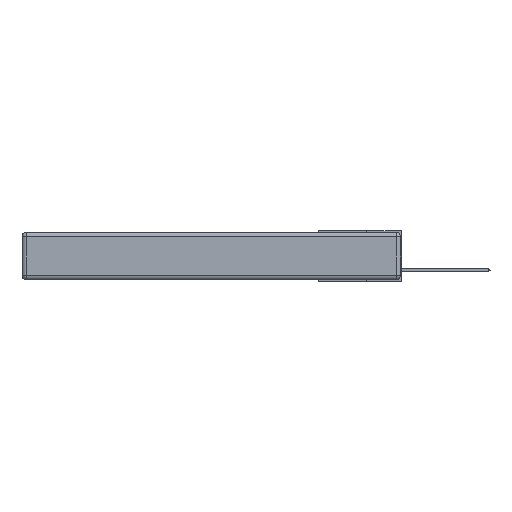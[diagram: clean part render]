
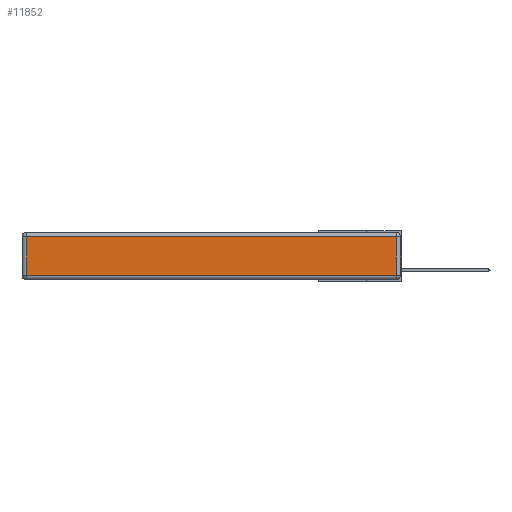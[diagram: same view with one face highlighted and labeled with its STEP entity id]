
A CAD part, left-side view. The second image highlights one B-rep face of the part: STEP entity #11852.
In plain terms, the highlighted planar face has unit normal (-1, 0, 0).
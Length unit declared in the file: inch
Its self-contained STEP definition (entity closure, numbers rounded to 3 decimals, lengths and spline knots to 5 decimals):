
#1438 = DIRECTION ( 'NONE',  ( -1., 0., 0. ) ) ;
#1815 = CARTESIAN_POINT ( 'NONE',  ( 0., 0.03, -0.03 ) ) ;
#3836 = CARTESIAN_POINT ( 'NONE',  ( 0., 2.72, -0.03 ) ) ;
#4516 = AXIS2_PLACEMENT_3D ( 'NONE', #21869, #1438, #6058 ) ;
#5223 = VECTOR ( 'NONE', #24640, 39.37008 ) ;
#5563 = VECTOR ( 'NONE', #8861, 39.37008 ) ;
#6058 = DIRECTION ( 'NONE',  ( 0., 0., 1. ) ) ;
#6269 = EDGE_CURVE ( 'NONE', #11951, #9548, #9448, .T. ) ;
#7486 = EDGE_CURVE ( 'NONE', #9548, #22008, #10480, .T. ) ;
#8087 = VERTEX_POINT ( 'NONE', #26164 ) ;
#8861 = DIRECTION ( 'NONE',  ( 0., -1., 0. ) ) ;
#9054 = CARTESIAN_POINT ( 'NONE',  ( 0., 2.75, -0.03 ) ) ;
#9448 = LINE ( 'NONE', #9054, #5223 ) ;
#9548 = VERTEX_POINT ( 'NONE', #3836 ) ;
#9661 = DIRECTION ( 'NONE',  ( 0., 0., 1. ) ) ;
#10480 = LINE ( 'NONE', #14195, #13611 ) ;
#11553 = LINE ( 'NONE', #27407, #26980 ) ;
#11852 = ADVANCED_FACE ( 'NONE', ( #28037 ), #19731, .T. ) ;
#11951 = VERTEX_POINT ( 'NONE', #1815 ) ;
#13611 = VECTOR ( 'NONE', #18722, 39.37008 ) ;
#13724 = ORIENTED_EDGE ( 'NONE', *, *, #7486, .T. ) ;
#14195 = CARTESIAN_POINT ( 'NONE',  ( 0., 2.72, -0.343 ) ) ;
#16173 = ORIENTED_EDGE ( 'NONE', *, *, #25970, .T. ) ;
#17398 = ORIENTED_EDGE ( 'NONE', *, *, #17653, .T. ) ;
#17653 = EDGE_CURVE ( 'NONE', #22008, #8087, #26604, .T. ) ;
#18722 = DIRECTION ( 'NONE',  ( 0., 0., -1. ) ) ;
#19731 = PLANE ( 'NONE',  #4516 ) ;
#21869 = CARTESIAN_POINT ( 'NONE',  ( 0., 0., -0.343 ) ) ;
#22008 = VERTEX_POINT ( 'NONE', #28251 ) ;
#23310 = ORIENTED_EDGE ( 'NONE', *, *, #6269, .T. ) ;
#24640 = DIRECTION ( 'NONE',  ( 0., 1., 0. ) ) ;
#25970 = EDGE_CURVE ( 'NONE', #8087, #11951, #11553, .T. ) ;
#26164 = CARTESIAN_POINT ( 'NONE',  ( 0., 0.03, -0.313 ) ) ;
#26323 = EDGE_LOOP ( 'NONE', ( #17398, #16173, #23310, #13724 ) ) ;
#26604 = LINE ( 'NONE', #28872, #5563 ) ;
#26980 = VECTOR ( 'NONE', #9661, 39.37008 ) ;
#27407 = CARTESIAN_POINT ( 'NONE',  ( 0., 0.03, -0.343 ) ) ;
#28037 = FACE_OUTER_BOUND ( 'NONE', #26323, .T. ) ;
#28251 = CARTESIAN_POINT ( 'NONE',  ( 0., 2.72, -0.313 ) ) ;
#28872 = CARTESIAN_POINT ( 'NONE',  ( 0., 0., -0.313 ) ) ;
